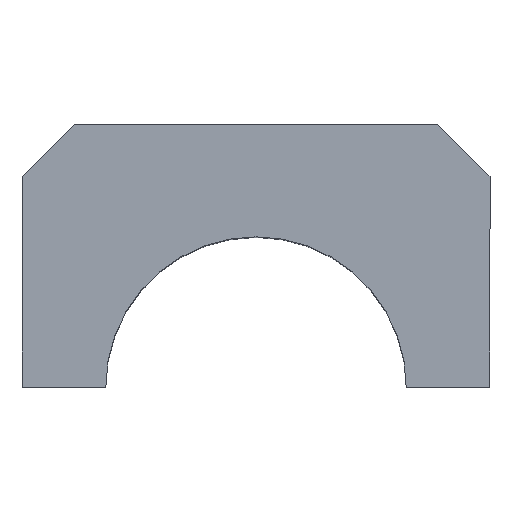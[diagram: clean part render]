
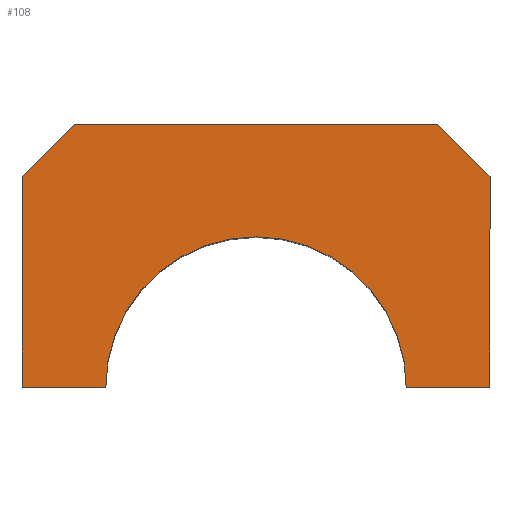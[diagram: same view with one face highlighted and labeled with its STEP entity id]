
A CAD part, top view. The second image highlights one B-rep face of the part: STEP entity #108.
In plain terms, the highlighted planar face has unit normal (0, 0, 1).
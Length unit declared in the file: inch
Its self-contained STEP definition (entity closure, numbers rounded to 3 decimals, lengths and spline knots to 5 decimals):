
#4 = CARTESIAN_POINT ( 'NONE',  ( 0., 0., 3.5 ) ) ;
#34 = LINE ( 'NONE', #602, #435 ) ;
#35 = AXIS2_PLACEMENT_3D ( 'NONE', #4, #142, #584 ) ;
#36 = CARTESIAN_POINT ( 'NONE',  ( 2.12248, 2.12248, 3.5 ) ) ;
#42 = VECTOR ( 'NONE', #168, 39.37008 ) ;
#45 = VERTEX_POINT ( 'NONE', #820 ) ;
#64 = VECTOR ( 'NONE', #360, 39.37008 ) ;
#68 = DIRECTION ( 'NONE',  ( 1., 0., 0. ) ) ;
#81 = ORIENTED_EDGE ( 'NONE', *, *, #368, .T. ) ;
#82 = ORIENTED_EDGE ( 'NONE', *, *, #766, .F. ) ;
#108 = ADVANCED_FACE ( 'NONE', ( #208 ), #522, .T. ) ;
#115 = VERTEX_POINT ( 'NONE', #456 ) ;
#124 = VERTEX_POINT ( 'NONE', #263 ) ;
#131 = CARTESIAN_POINT ( 'NONE',  ( 1.435, 0., 3.5 ) ) ;
#142 = DIRECTION ( 'NONE',  ( 0., 0., 1. ) ) ;
#153 = CARTESIAN_POINT ( 'NONE',  ( -1.735, 2.50996, 3.5 ) ) ;
#158 = CARTESIAN_POINT ( 'NONE',  ( -2.235, 0., 3.5 ) ) ;
#160 = VERTEX_POINT ( 'NONE', #131 ) ;
#168 = DIRECTION ( 'NONE',  ( 0., 1., 0. ) ) ;
#185 = EDGE_CURVE ( 'NONE', #798, #124, #710, .T. ) ;
#189 = VECTOR ( 'NONE', #661, 39.37008 ) ;
#207 = VERTEX_POINT ( 'NONE', #271 ) ;
#208 = FACE_OUTER_BOUND ( 'NONE', #643, .T. ) ;
#234 = VECTOR ( 'NONE', #471, 39.37008 ) ;
#256 = CARTESIAN_POINT ( 'NONE',  ( -1.435, 0., 3.5 ) ) ;
#263 = CARTESIAN_POINT ( 'NONE',  ( -2.235, 2.00996, 3.5 ) ) ;
#264 = LINE ( 'NONE', #822, #42 ) ;
#271 = CARTESIAN_POINT ( 'NONE',  ( -2.235, 0., 3.5 ) ) ;
#286 = VERTEX_POINT ( 'NONE', #530 ) ;
#291 = AXIS2_PLACEMENT_3D ( 'NONE', #628, #451, #68 ) ;
#293 = VECTOR ( 'NONE', #673, 39.37008 ) ;
#302 = LINE ( 'NONE', #158, #293 ) ;
#316 = CIRCLE ( 'NONE', #291, 1.435 ) ;
#353 = LINE ( 'NONE', #36, #64 ) ;
#360 = DIRECTION ( 'NONE',  ( -0.707, 0.707, 0. ) ) ;
#368 = EDGE_CURVE ( 'NONE', #286, #798, #34, .T. ) ;
#371 = ORIENTED_EDGE ( 'NONE', *, *, #185, .T. ) ;
#406 = LINE ( 'NONE', #479, #234 ) ;
#408 = CARTESIAN_POINT ( 'NONE',  ( -2.12248, 2.12248, 3.5 ) ) ;
#435 = VECTOR ( 'NONE', #606, 39.37008 ) ;
#450 = ORIENTED_EDGE ( 'NONE', *, *, #741, .T. ) ;
#451 = DIRECTION ( 'NONE',  ( 0., 0., 1. ) ) ;
#456 = CARTESIAN_POINT ( 'NONE',  ( 2.235, 2.00996, 3.5 ) ) ;
#471 = DIRECTION ( 'NONE',  ( -1., 0., 0. ) ) ;
#473 = VECTOR ( 'NONE', #567, 39.37008 ) ;
#479 = CARTESIAN_POINT ( 'NONE',  ( 0., 0., 3.5 ) ) ;
#502 = ORIENTED_EDGE ( 'NONE', *, *, #589, .T. ) ;
#522 = PLANE ( 'NONE',  #35 ) ;
#530 = CARTESIAN_POINT ( 'NONE',  ( 1.735, 2.50996, 3.5 ) ) ;
#531 = EDGE_CURVE ( 'NONE', #45, #115, #264, .T. ) ;
#567 = DIRECTION ( 'NONE',  ( 1., 0., 0. ) ) ;
#584 = DIRECTION ( 'NONE',  ( 1., 0., 0. ) ) ;
#589 = EDGE_CURVE ( 'NONE', #115, #286, #353, .T. ) ;
#602 = CARTESIAN_POINT ( 'NONE',  ( 0., 2.50996, 3.5 ) ) ;
#606 = DIRECTION ( 'NONE',  ( -1., 0., 0. ) ) ;
#626 = CARTESIAN_POINT ( 'NONE',  ( 0., 0., 3.5 ) ) ;
#628 = CARTESIAN_POINT ( 'NONE',  ( 0., 0., 3.5 ) ) ;
#643 = EDGE_LOOP ( 'NONE', ( #81, #371, #450, #82, #796, #720, #764, #502 ) ) ;
#661 = DIRECTION ( 'NONE',  ( -0.707, -0.707, 0. ) ) ;
#669 = EDGE_CURVE ( 'NONE', #160, #686, #316, .T. ) ;
#673 = DIRECTION ( 'NONE',  ( 0., -1., 0. ) ) ;
#677 = EDGE_CURVE ( 'NONE', #160, #45, #825, .T. ) ;
#686 = VERTEX_POINT ( 'NONE', #256 ) ;
#710 = LINE ( 'NONE', #408, #189 ) ;
#720 = ORIENTED_EDGE ( 'NONE', *, *, #677, .T. ) ;
#741 = EDGE_CURVE ( 'NONE', #124, #207, #302, .T. ) ;
#764 = ORIENTED_EDGE ( 'NONE', *, *, #531, .T. ) ;
#766 = EDGE_CURVE ( 'NONE', #686, #207, #406, .T. ) ;
#796 = ORIENTED_EDGE ( 'NONE', *, *, #669, .F. ) ;
#798 = VERTEX_POINT ( 'NONE', #153 ) ;
#820 = CARTESIAN_POINT ( 'NONE',  ( 2.235, 0., 3.5 ) ) ;
#822 = CARTESIAN_POINT ( 'NONE',  ( 2.235, 0., 3.5 ) ) ;
#825 = LINE ( 'NONE', #626, #473 ) ;
